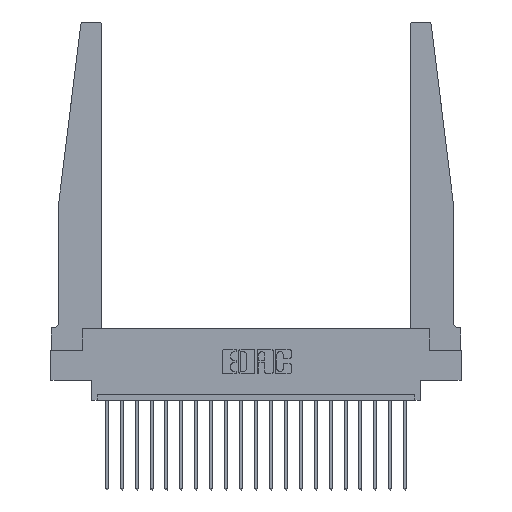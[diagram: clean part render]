
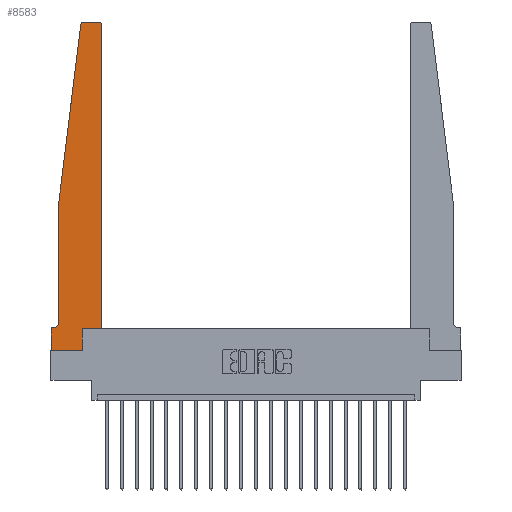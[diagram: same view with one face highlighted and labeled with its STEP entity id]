
A CAD part, top view. The second image highlights one B-rep face of the part: STEP entity #8583.
In plain terms, the highlighted planar face has unit normal (0, 0, 1).
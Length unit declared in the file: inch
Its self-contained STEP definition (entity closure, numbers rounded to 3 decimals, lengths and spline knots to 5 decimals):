
#252 = ORIENTED_EDGE ( 'NONE', *, *, #376, .T. ) ;
#376 = EDGE_CURVE ( 'NONE', #499, #9541, #15689, .T. ) ;
#484 = DIRECTION ( 'NONE',  ( -1., 0., 0. ) ) ;
#499 = VERTEX_POINT ( 'NONE', #17385 ) ;
#654 = DIRECTION ( 'NONE',  ( -1., 0., 0. ) ) ;
#950 = CARTESIAN_POINT ( 'NONE',  ( 0.065, 0.2375, 0.37 ) ) ;
#1231 = EDGE_CURVE ( 'NONE', #15519, #13941, #11612, .T. ) ;
#1516 = VERTEX_POINT ( 'NONE', #2307 ) ;
#1661 = AXIS2_PLACEMENT_3D ( 'NONE', #17834, #17733, #14413 ) ;
#1684 = VERTEX_POINT ( 'NONE', #11075 ) ;
#1910 = EDGE_CURVE ( 'NONE', #14734, #9078, #18885, .T. ) ;
#1991 = CARTESIAN_POINT ( 'NONE',  ( 0.25, 2.75, 0.37 ) ) ;
#2071 = VERTEX_POINT ( 'NONE', #19095 ) ;
#2307 = CARTESIAN_POINT ( 'NONE',  ( 0., 0.1875, 0.37 ) ) ;
#2314 = LINE ( 'NONE', #1991, #3624 ) ;
#3108 = EDGE_CURVE ( 'NONE', #6056, #10813, #17024, .T. ) ;
#3181 = AXIS2_PLACEMENT_3D ( 'NONE', #14504, #20857, #21066 ) ;
#3257 = CIRCLE ( 'NONE', #8749, 0.05 ) ;
#3285 = ORIENTED_EDGE ( 'NONE', *, *, #6369, .T. ) ;
#3326 = ORIENTED_EDGE ( 'NONE', *, *, #1910, .T. ) ;
#3431 = EDGE_CURVE ( 'NONE', #2071, #15519, #2314, .T. ) ;
#3438 = VECTOR ( 'NONE', #7098, 39.37008 ) ;
#3624 = VECTOR ( 'NONE', #484, 39.37008 ) ;
#4064 = LINE ( 'NONE', #6984, #11456 ) ;
#4514 = EDGE_CURVE ( 'NONE', #13941, #14734, #19367, .T. ) ;
#4680 = CARTESIAN_POINT ( 'NONE',  ( 0.065, 1.25, 0.37 ) ) ;
#5096 = CARTESIAN_POINT ( 'NONE',  ( 0.425, 2.72, 0.37 ) ) ;
#5706 = DIRECTION ( 'NONE',  ( 0., 0., 1. ) ) ;
#5736 = DIRECTION ( 'NONE',  ( 0., 1., 0. ) ) ;
#6039 = CARTESIAN_POINT ( 'NONE',  ( 0., 0., 0.37 ) ) ;
#6056 = VERTEX_POINT ( 'NONE', #7880 ) ;
#6369 = EDGE_CURVE ( 'NONE', #1516, #6056, #20530, .T. ) ;
#6424 = VERTEX_POINT ( 'NONE', #20731 ) ;
#6984 = CARTESIAN_POINT ( 'NONE',  ( 0.065, 0.1875, 0.37 ) ) ;
#7098 = DIRECTION ( 'NONE',  ( 1., 0., 0. ) ) ;
#7100 = AXIS2_PLACEMENT_3D ( 'NONE', #20403, #5706, #17565 ) ;
#7323 = PLANE ( 'NONE',  #7100 ) ;
#7805 = EDGE_CURVE ( 'NONE', #6424, #1516, #4064, .T. ) ;
#7880 = CARTESIAN_POINT ( 'NONE',  ( 0., 0., 0.37 ) ) ;
#8262 = LINE ( 'NONE', #11153, #17881 ) ;
#8583 = ADVANCED_FACE ( 'NONE', ( #15454 ), #7323, .T. ) ;
#8749 = AXIS2_PLACEMENT_3D ( 'NONE', #10628, #20182, #654 ) ;
#8984 = CARTESIAN_POINT ( 'NONE',  ( 0., 0., 0.37 ) ) ;
#9078 = VERTEX_POINT ( 'NONE', #950 ) ;
#9541 = VERTEX_POINT ( 'NONE', #5096 ) ;
#10144 = EDGE_CURVE ( 'NONE', #1684, #499, #13834, .T. ) ;
#10165 = EDGE_LOOP ( 'NONE', ( #10239, #14516, #12949, #3326, #12191, #15957, #3285, #14356, #17823, #14267, #252, #17841 ) ) ;
#10239 = ORIENTED_EDGE ( 'NONE', *, *, #3431, .T. ) ;
#10343 = CARTESIAN_POINT ( 'NONE',  ( 0.27653, 2.75, 0.37 ) ) ;
#10347 = CARTESIAN_POINT ( 'NONE',  ( 0.24675, 2.72367, 0.37 ) ) ;
#10628 = CARTESIAN_POINT ( 'NONE',  ( 0.015, 0.2375, 0.37 ) ) ;
#10813 = VERTEX_POINT ( 'NONE', #14013 ) ;
#11075 = CARTESIAN_POINT ( 'NONE',  ( 0.2605, 0.18, 0.37 ) ) ;
#11153 = CARTESIAN_POINT ( 'NONE',  ( 0.2605, 0.18, 0.37 ) ) ;
#11222 = DIRECTION ( 'NONE',  ( -0.122, -0.992, 0. ) ) ;
#11456 = VECTOR ( 'NONE', #20269, 39.37008 ) ;
#11612 = CIRCLE ( 'NONE', #1661, 0.03 ) ;
#12038 = CARTESIAN_POINT ( 'NONE',  ( 0.065, 1.25, 0.37 ) ) ;
#12191 = ORIENTED_EDGE ( 'NONE', *, *, #19725, .T. ) ;
#12664 = VECTOR ( 'NONE', #20197, 39.37008 ) ;
#12949 = ORIENTED_EDGE ( 'NONE', *, *, #4514, .T. ) ;
#13834 = LINE ( 'NONE', #15434, #3438 ) ;
#13876 = CARTESIAN_POINT ( 'NONE',  ( 0.425, 0.18, 0.37 ) ) ;
#13941 = VERTEX_POINT ( 'NONE', #10347 ) ;
#14013 = CARTESIAN_POINT ( 'NONE',  ( 0.2605, 0., 0.37 ) ) ;
#14267 = ORIENTED_EDGE ( 'NONE', *, *, #10144, .T. ) ;
#14356 = ORIENTED_EDGE ( 'NONE', *, *, #3108, .T. ) ;
#14405 = VECTOR ( 'NONE', #11222, 39.37008 ) ;
#14413 = DIRECTION ( 'NONE',  ( 1., 0., 0. ) ) ;
#14504 = CARTESIAN_POINT ( 'NONE',  ( 0.395, 2.72, 0.37 ) ) ;
#14516 = ORIENTED_EDGE ( 'NONE', *, *, #1231, .T. ) ;
#14523 = EDGE_CURVE ( 'NONE', #10813, #1684, #8262, .T. ) ;
#14734 = VERTEX_POINT ( 'NONE', #14890 ) ;
#14890 = CARTESIAN_POINT ( 'NONE',  ( 0.065, 1.25, 0.37 ) ) ;
#15169 = EDGE_CURVE ( 'NONE', #9541, #2071, #20335, .T. ) ;
#15434 = CARTESIAN_POINT ( 'NONE',  ( 0.425, 0.18, 0.37 ) ) ;
#15454 = FACE_OUTER_BOUND ( 'NONE', #10165, .T. ) ;
#15519 = VERTEX_POINT ( 'NONE', #10343 ) ;
#15689 = LINE ( 'NONE', #13876, #17064 ) ;
#15957 = ORIENTED_EDGE ( 'NONE', *, *, #7805, .T. ) ;
#17024 = LINE ( 'NONE', #8984, #19698 ) ;
#17064 = VECTOR ( 'NONE', #5736, 39.37008 ) ;
#17385 = CARTESIAN_POINT ( 'NONE',  ( 0.425, 0.18, 0.37 ) ) ;
#17565 = DIRECTION ( 'NONE',  ( 1., 0., 0. ) ) ;
#17733 = DIRECTION ( 'NONE',  ( 0., 0., 1. ) ) ;
#17823 = ORIENTED_EDGE ( 'NONE', *, *, #14523, .T. ) ;
#17834 = CARTESIAN_POINT ( 'NONE',  ( 0.27653, 2.72, 0.37 ) ) ;
#17841 = ORIENTED_EDGE ( 'NONE', *, *, #15169, .T. ) ;
#17881 = VECTOR ( 'NONE', #19298, 39.37008 ) ;
#18885 = LINE ( 'NONE', #12038, #12664 ) ;
#19003 = DIRECTION ( 'NONE',  ( 0., -1., 0. ) ) ;
#19095 = CARTESIAN_POINT ( 'NONE',  ( 0.395, 2.75, 0.37 ) ) ;
#19298 = DIRECTION ( 'NONE',  ( 0., 1., 0. ) ) ;
#19367 = LINE ( 'NONE', #4680, #14405 ) ;
#19698 = VECTOR ( 'NONE', #20152, 39.37008 ) ;
#19725 = EDGE_CURVE ( 'NONE', #9078, #6424, #3257, .T. ) ;
#20152 = DIRECTION ( 'NONE',  ( 1., 0., 0. ) ) ;
#20182 = DIRECTION ( 'NONE',  ( 0., 0., -1. ) ) ;
#20197 = DIRECTION ( 'NONE',  ( 0., -1., 0. ) ) ;
#20269 = DIRECTION ( 'NONE',  ( -1., 0., 0. ) ) ;
#20335 = CIRCLE ( 'NONE', #3181, 0.03 ) ;
#20403 = CARTESIAN_POINT ( 'NONE',  ( 0., 0.1875, 0.37 ) ) ;
#20530 = LINE ( 'NONE', #6039, #21192 ) ;
#20731 = CARTESIAN_POINT ( 'NONE',  ( 0.015, 0.1875, 0.37 ) ) ;
#20857 = DIRECTION ( 'NONE',  ( 0., 0., 1. ) ) ;
#21066 = DIRECTION ( 'NONE',  ( 1., 0., 0. ) ) ;
#21192 = VECTOR ( 'NONE', #19003, 39.37008 ) ;
